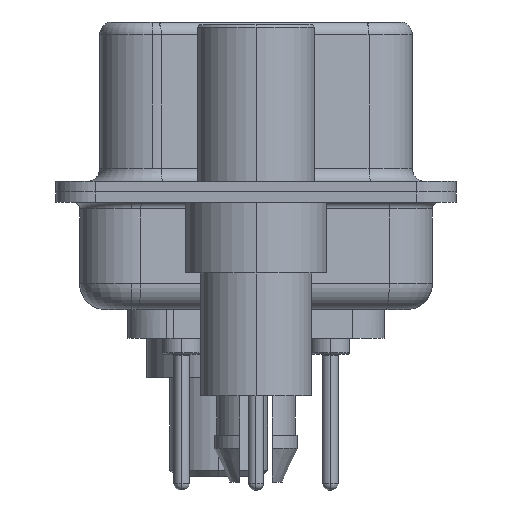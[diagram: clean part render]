
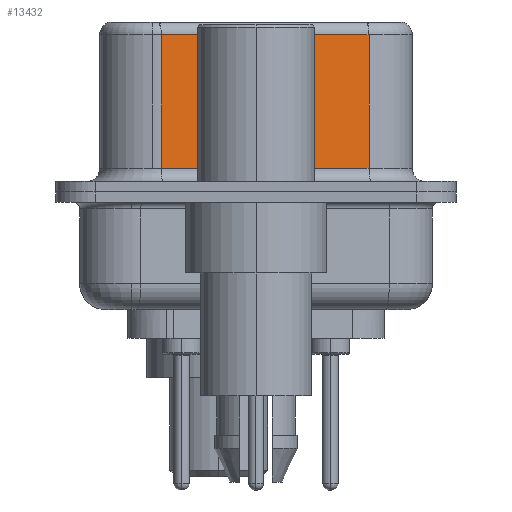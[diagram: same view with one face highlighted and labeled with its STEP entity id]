
A CAD part, left-side view. The second image highlights one B-rep face of the part: STEP entity #13432.
In plain terms, the highlighted planar face has unit normal (-0.985, -0.174, 0).
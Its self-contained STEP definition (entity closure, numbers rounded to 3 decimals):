
#870 = EDGE_LOOP ( 'NONE', ( #12416, #6472, #17240, #29802 ) ) ;
#999 = DIRECTION ( 'NONE',  ( 0., 0., -1. ) ) ;
#1786 = LINE ( 'NONE', #26434, #18285 ) ;
#2005 = DIRECTION ( 'NONE',  ( 0., 0., -1. ) ) ;
#3937 = VECTOR ( 'NONE', #30458, 1000. ) ;
#4973 = CARTESIAN_POINT ( 'NONE',  ( 3.73, 3.628, 6.02 ) ) ;
#5939 = CARTESIAN_POINT ( 'NONE',  ( 5.132, -4.322, 6.02 ) ) ;
#6472 = ORIENTED_EDGE ( 'NONE', *, *, #8782, .T. ) ;
#6906 = DIRECTION ( 'NONE',  ( 0.985, 0.174, 0. ) ) ;
#8782 = EDGE_CURVE ( 'NONE', #23259, #16557, #22702, .T. ) ;
#10624 = LINE ( 'NONE', #18197, #24406 ) ;
#10871 = VERTEX_POINT ( 'NONE', #28871 ) ;
#12416 = ORIENTED_EDGE ( 'NONE', *, *, #25322, .F. ) ;
#13432 = ADVANCED_FACE ( 'NONE', ( #15028 ), #31394, .F. ) ;
#14570 = DIRECTION ( 'NONE',  ( 0.174, -0.985, 0. ) ) ;
#15028 = FACE_OUTER_BOUND ( 'NONE', #870, .T. ) ;
#16495 = EDGE_CURVE ( 'NONE', #18900, #10871, #25183, .T. ) ;
#16557 = VERTEX_POINT ( 'NONE', #4973 ) ;
#17240 = ORIENTED_EDGE ( 'NONE', *, *, #25508, .T. ) ;
#18197 = CARTESIAN_POINT ( 'NONE',  ( 5.132, -4.322, 6.52 ) ) ;
#18285 = VECTOR ( 'NONE', #2005, 1000. ) ;
#18698 = VECTOR ( 'NONE', #14570, 1000. ) ;
#18900 = VERTEX_POINT ( 'NONE', #31696 ) ;
#19128 = CARTESIAN_POINT ( 'NONE',  ( 5.132, -4.322, 6.52 ) ) ;
#21826 = CARTESIAN_POINT ( 'NONE',  ( 5.132, -4.322, 0.9 ) ) ;
#22686 = AXIS2_PLACEMENT_3D ( 'NONE', #19128, #6906, #24035 ) ;
#22702 = LINE ( 'NONE', #5939, #3937 ) ;
#23259 = VERTEX_POINT ( 'NONE', #28930 ) ;
#24035 = DIRECTION ( 'NONE',  ( -0.174, 0.985, 0. ) ) ;
#24406 = VECTOR ( 'NONE', #999, 1000. ) ;
#25183 = LINE ( 'NONE', #21826, #18698 ) ;
#25322 = EDGE_CURVE ( 'NONE', #23259, #10871, #10624, .T. ) ;
#25508 = EDGE_CURVE ( 'NONE', #16557, #18900, #1786, .T. ) ;
#26434 = CARTESIAN_POINT ( 'NONE',  ( 3.73, 3.628, 6.52 ) ) ;
#28871 = CARTESIAN_POINT ( 'NONE',  ( 5.132, -4.322, 0.9 ) ) ;
#28930 = CARTESIAN_POINT ( 'NONE',  ( 5.132, -4.322, 6.02 ) ) ;
#29802 = ORIENTED_EDGE ( 'NONE', *, *, #16495, .T. ) ;
#30458 = DIRECTION ( 'NONE',  ( -0.174, 0.985, 0. ) ) ;
#31394 = PLANE ( 'NONE',  #22686 ) ;
#31696 = CARTESIAN_POINT ( 'NONE',  ( 3.73, 3.628, 0.9 ) ) ;
